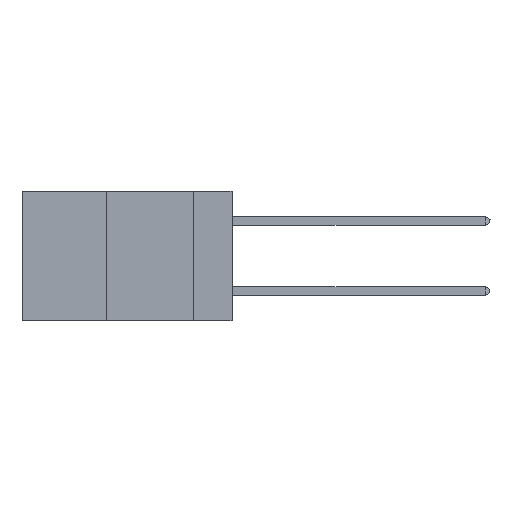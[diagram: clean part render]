
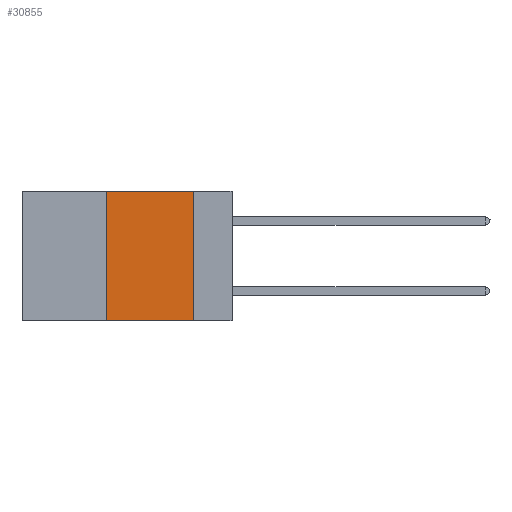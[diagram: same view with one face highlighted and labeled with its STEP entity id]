
A CAD part, left-side view. The second image highlights one B-rep face of the part: STEP entity #30855.
In plain terms, the highlighted planar face has unit normal (-1, 0, 0).
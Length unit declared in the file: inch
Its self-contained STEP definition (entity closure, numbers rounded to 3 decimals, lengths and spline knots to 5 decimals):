
#3060 = PLANE ( 'NONE',  #28158 ) ;
#3891 = CARTESIAN_POINT ( 'NONE',  ( 0., 0.6, -0.37 ) ) ;
#5776 = ORIENTED_EDGE ( 'NONE', *, *, #22018, .F. ) ;
#7165 = CARTESIAN_POINT ( 'NONE',  ( 0., 0.11, 0. ) ) ;
#8145 = CARTESIAN_POINT ( 'NONE',  ( 0., 0.11, 0. ) ) ;
#8540 = LINE ( 'NONE', #8145, #15848 ) ;
#10619 = ORIENTED_EDGE ( 'NONE', *, *, #28069, .F. ) ;
#11545 = EDGE_CURVE ( 'NONE', #16975, #20920, #33070, .T. ) ;
#12323 = LINE ( 'NONE', #21651, #34214 ) ;
#14131 = DIRECTION ( 'NONE',  ( 0., 0., 1. ) ) ;
#14239 = DIRECTION ( 'NONE',  ( 0., 0., -1. ) ) ;
#14772 = CARTESIAN_POINT ( 'NONE',  ( 0., 0.36, -0.37 ) ) ;
#15793 = VERTEX_POINT ( 'NONE', #15930 ) ;
#15848 = VECTOR ( 'NONE', #38509, 39.37008 ) ;
#15930 = CARTESIAN_POINT ( 'NONE',  ( 0., 0.36, 0. ) ) ;
#16975 = VERTEX_POINT ( 'NONE', #14772 ) ;
#18955 = DIRECTION ( 'NONE',  ( 0., -1., 0. ) ) ;
#20920 = VERTEX_POINT ( 'NONE', #25592 ) ;
#21651 = CARTESIAN_POINT ( 'NONE',  ( 0., 0.6, 0. ) ) ;
#22018 = EDGE_CURVE ( 'NONE', #15793, #31468, #12323, .T. ) ;
#24082 = CARTESIAN_POINT ( 'NONE',  ( 0., 0.6, 0. ) ) ;
#25443 = CARTESIAN_POINT ( 'NONE',  ( 0., 0.36, 0. ) ) ;
#25592 = CARTESIAN_POINT ( 'NONE',  ( 0., 0.11, -0.37 ) ) ;
#27275 = EDGE_LOOP ( 'NONE', ( #10619, #5776, #34785, #38811 ) ) ;
#28069 = EDGE_CURVE ( 'NONE', #31468, #20920, #8540, .T. ) ;
#28158 = AXIS2_PLACEMENT_3D ( 'NONE', #24082, #29119, #14239 ) ;
#29119 = DIRECTION ( 'NONE',  ( 1., 0., 0. ) ) ;
#29734 = EDGE_CURVE ( 'NONE', #16975, #15793, #35167, .T. ) ;
#30855 = ADVANCED_FACE ( 'NONE', ( #38455 ), #3060, .F. ) ;
#31468 = VERTEX_POINT ( 'NONE', #7165 ) ;
#31776 = VECTOR ( 'NONE', #14131, 39.37008 ) ;
#33070 = LINE ( 'NONE', #3891, #36859 ) ;
#34214 = VECTOR ( 'NONE', #36543, 39.37008 ) ;
#34785 = ORIENTED_EDGE ( 'NONE', *, *, #29734, .F. ) ;
#35167 = LINE ( 'NONE', #25443, #31776 ) ;
#36543 = DIRECTION ( 'NONE',  ( 0., -1., 0. ) ) ;
#36859 = VECTOR ( 'NONE', #18955, 39.37008 ) ;
#38455 = FACE_OUTER_BOUND ( 'NONE', #27275, .T. ) ;
#38509 = DIRECTION ( 'NONE',  ( 0., 0., -1. ) ) ;
#38811 = ORIENTED_EDGE ( 'NONE', *, *, #11545, .T. ) ;
